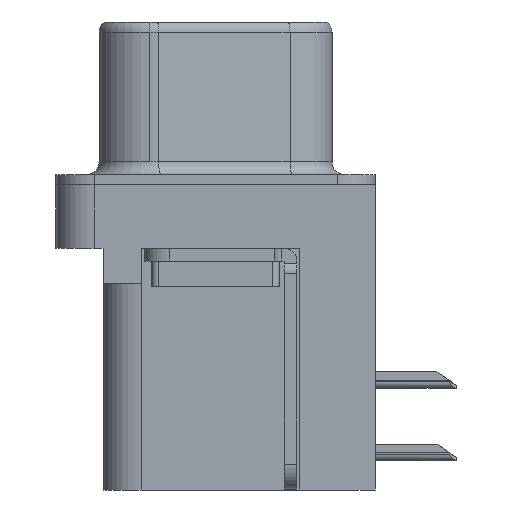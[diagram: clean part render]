
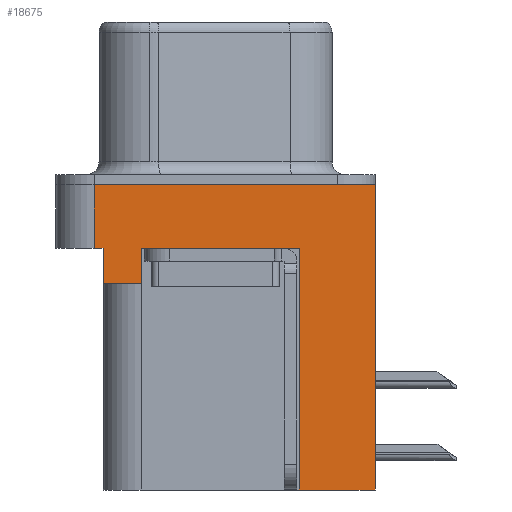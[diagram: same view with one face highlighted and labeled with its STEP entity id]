
A CAD part, left-side view. The second image highlights one B-rep face of the part: STEP entity #18675.
In plain terms, the highlighted planar face has unit normal (-1, 0, 0).
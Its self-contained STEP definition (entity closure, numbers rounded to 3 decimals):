
#150 = ORIENTED_EDGE ( 'NONE', *, *, #19896, .F. ) ;
#650 = ORIENTED_EDGE ( 'NONE', *, *, #9167, .F. ) ;
#1540 = LINE ( 'NONE', #22992, #13706 ) ;
#1567 = DIRECTION ( 'NONE',  ( 0., 0., 1. ) ) ;
#1680 = DIRECTION ( 'NONE',  ( 0., -1., 0. ) ) ;
#2813 = VECTOR ( 'NONE', #7578, 1000. ) ;
#2991 = VECTOR ( 'NONE', #1680, 1000. ) ;
#3354 = VERTEX_POINT ( 'NONE', #12885 ) ;
#3610 = VERTEX_POINT ( 'NONE', #19283 ) ;
#4144 = DIRECTION ( 'NONE',  ( 0., 0., 1. ) ) ;
#4182 = VECTOR ( 'NONE', #4144, 1000. ) ;
#4365 = VERTEX_POINT ( 'NONE', #24288 ) ;
#4994 = CARTESIAN_POINT ( 'NONE',  ( -2.91, -6.275, -2.5 ) ) ;
#5561 = DIRECTION ( 'NONE',  ( 0., 0., 1. ) ) ;
#5887 = DIRECTION ( 'NONE',  ( 0., 1., 0. ) ) ;
#6585 = VECTOR ( 'NONE', #5887, 1000. ) ;
#6829 = EDGE_CURVE ( 'NONE', #9145, #3610, #24289, .T. ) ;
#6905 = ORIENTED_EDGE ( 'NONE', *, *, #16365, .F. ) ;
#6979 = CARTESIAN_POINT ( 'NONE',  ( -2.91, 4.425, -3.9 ) ) ;
#6985 = PLANE ( 'NONE',  #14859 ) ;
#7064 = DIRECTION ( 'NONE',  ( 0., 1., 0. ) ) ;
#7246 = ORIENTED_EDGE ( 'NONE', *, *, #18756, .T. ) ;
#7392 = CARTESIAN_POINT ( 'NONE',  ( -2.91, 4.425, -3.9 ) ) ;
#7560 = LINE ( 'NONE', #8133, #14695 ) ;
#7578 = DIRECTION ( 'NONE',  ( 0., -1., 0. ) ) ;
#7925 = CARTESIAN_POINT ( 'NONE',  ( -2.91, -6.275, 0. ) ) ;
#8133 = CARTESIAN_POINT ( 'NONE',  ( -2.91, -6.275, -2.5 ) ) ;
#8644 = LINE ( 'NONE', #18980, #17591 ) ;
#8690 = VERTEX_POINT ( 'NONE', #12019 ) ;
#9046 = LINE ( 'NONE', #6979, #17938 ) ;
#9048 = CARTESIAN_POINT ( 'NONE',  ( -2.91, 4.425, -2.5 ) ) ;
#9145 = VERTEX_POINT ( 'NONE', #10698 ) ;
#9167 = EDGE_CURVE ( 'NONE', #12908, #14712, #14475, .T. ) ;
#9247 = ORIENTED_EDGE ( 'NONE', *, *, #11609, .F. ) ;
#9850 = DIRECTION ( 'NONE',  ( 0., -1., 0. ) ) ;
#10114 = VERTEX_POINT ( 'NONE', #14650 ) ;
#10698 = CARTESIAN_POINT ( 'NONE',  ( -2.91, 2.895, -2.5 ) ) ;
#10909 = CARTESIAN_POINT ( 'NONE',  ( -2.91, -6.275, -2.5 ) ) ;
#11049 = ORIENTED_EDGE ( 'NONE', *, *, #18984, .T. ) ;
#11609 = EDGE_CURVE ( 'NONE', #8690, #4365, #18471, .T. ) ;
#11757 = VERTEX_POINT ( 'NONE', #17767 ) ;
#12019 = CARTESIAN_POINT ( 'NONE',  ( -2.91, 4.775, 0. ) ) ;
#12681 = FACE_OUTER_BOUND ( 'NONE', #17018, .T. ) ;
#12775 = DIRECTION ( 'NONE',  ( -1., 0., 0. ) ) ;
#12791 = VERTEX_POINT ( 'NONE', #14257 ) ;
#12885 = CARTESIAN_POINT ( 'NONE',  ( -2.91, 4.775, -2.5 ) ) ;
#12908 = VERTEX_POINT ( 'NONE', #20526 ) ;
#12966 = LINE ( 'NONE', #22439, #2813 ) ;
#13386 = CARTESIAN_POINT ( 'NONE',  ( -2.91, 2.895, -3.9 ) ) ;
#13706 = VECTOR ( 'NONE', #21727, 1000. ) ;
#14257 = CARTESIAN_POINT ( 'NONE',  ( -2.91, -6.275, -12. ) ) ;
#14343 = VECTOR ( 'NONE', #9850, 1000. ) ;
#14475 = LINE ( 'NONE', #7392, #17987 ) ;
#14650 = CARTESIAN_POINT ( 'NONE',  ( -2.91, 2.895, -3.9 ) ) ;
#14695 = VECTOR ( 'NONE', #23208, 1000. ) ;
#14712 = VERTEX_POINT ( 'NONE', #9048 ) ;
#14859 = AXIS2_PLACEMENT_3D ( 'NONE', #4994, #12775, #1567 ) ;
#15540 = CARTESIAN_POINT ( 'NONE',  ( -2.91, -3.295, -12. ) ) ;
#16190 = ORIENTED_EDGE ( 'NONE', *, *, #18206, .F. ) ;
#16365 = EDGE_CURVE ( 'NONE', #11757, #3610, #8644, .T. ) ;
#17018 = EDGE_LOOP ( 'NONE', ( #9247, #23784, #7246, #650, #16190, #22945, #20898, #6905, #150, #11049 ) ) ;
#17591 = VECTOR ( 'NONE', #21242, 1000. ) ;
#17767 = CARTESIAN_POINT ( 'NONE',  ( -2.91, -3.295, -12. ) ) ;
#17938 = VECTOR ( 'NONE', #7064, 1000. ) ;
#17987 = VECTOR ( 'NONE', #5561, 1000. ) ;
#18206 = EDGE_CURVE ( 'NONE', #10114, #12908, #9046, .T. ) ;
#18471 = LINE ( 'NONE', #7925, #14343 ) ;
#18675 = ADVANCED_FACE ( 'NONE', ( #12681 ), #6985, .T. ) ;
#18756 = EDGE_CURVE ( 'NONE', #3354, #14712, #12966, .T. ) ;
#18980 = CARTESIAN_POINT ( 'NONE',  ( -2.91, -3.295, -12. ) ) ;
#18984 = EDGE_CURVE ( 'NONE', #12791, #4365, #7560, .T. ) ;
#19283 = CARTESIAN_POINT ( 'NONE',  ( -2.91, -3.295, -2.5 ) ) ;
#19896 = EDGE_CURVE ( 'NONE', #12791, #11757, #22258, .T. ) ;
#20526 = CARTESIAN_POINT ( 'NONE',  ( -2.91, 4.425, -3.9 ) ) ;
#20585 = EDGE_CURVE ( 'NONE', #10114, #9145, #21043, .T. ) ;
#20630 = EDGE_CURVE ( 'NONE', #3354, #8690, #1540, .T. ) ;
#20898 = ORIENTED_EDGE ( 'NONE', *, *, #6829, .T. ) ;
#21043 = LINE ( 'NONE', #13386, #4182 ) ;
#21242 = DIRECTION ( 'NONE',  ( 0., 0., 1. ) ) ;
#21727 = DIRECTION ( 'NONE',  ( 0., 0., 1. ) ) ;
#22258 = LINE ( 'NONE', #15540, #6585 ) ;
#22439 = CARTESIAN_POINT ( 'NONE',  ( -2.91, -6.275, -2.5 ) ) ;
#22945 = ORIENTED_EDGE ( 'NONE', *, *, #20585, .T. ) ;
#22992 = CARTESIAN_POINT ( 'NONE',  ( -2.91, 4.775, -2.5 ) ) ;
#23208 = DIRECTION ( 'NONE',  ( 0., 0., 1. ) ) ;
#23784 = ORIENTED_EDGE ( 'NONE', *, *, #20630, .F. ) ;
#24288 = CARTESIAN_POINT ( 'NONE',  ( -2.91, -6.275, 0. ) ) ;
#24289 = LINE ( 'NONE', #10909, #2991 ) ;
